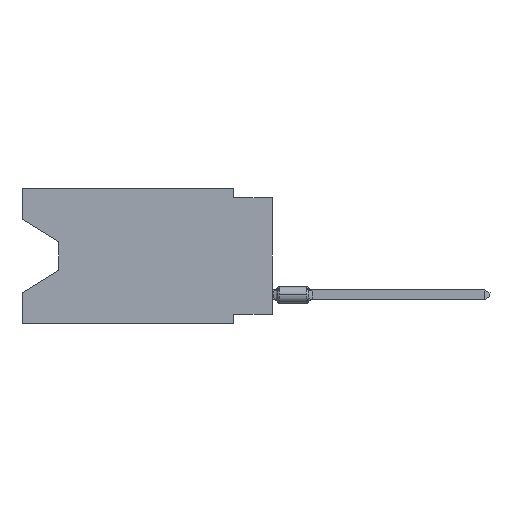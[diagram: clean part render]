
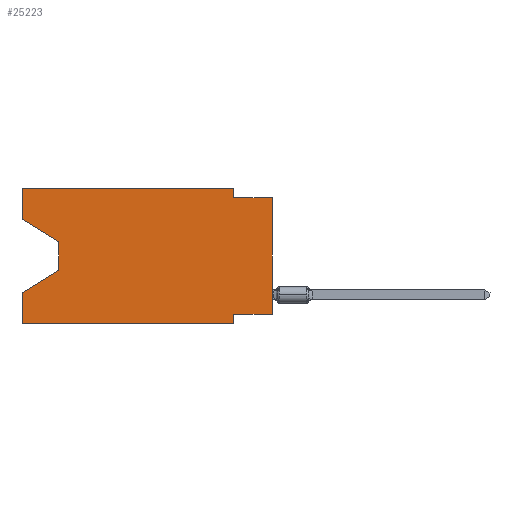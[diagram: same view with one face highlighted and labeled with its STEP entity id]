
A CAD part, left-side view. The second image highlights one B-rep face of the part: STEP entity #25223.
In plain terms, the highlighted planar face has unit normal (-1, 0, 0).
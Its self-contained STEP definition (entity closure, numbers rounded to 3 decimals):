
#1275 = EDGE_CURVE ( 'NONE', #24755, #3150, #7686, .T. ) ;
#1803 = CARTESIAN_POINT ( 'NONE',  ( 0., 16.383, -8.89 ) ) ;
#1833 = VECTOR ( 'NONE', #9087, 1000. ) ;
#2582 = VERTEX_POINT ( 'NONE', #27055 ) ;
#2785 = VECTOR ( 'NONE', #10349, 1000. ) ;
#3089 = EDGE_CURVE ( 'NONE', #15983, #5152, #23669, .T. ) ;
#3150 = VERTEX_POINT ( 'NONE', #28133 ) ;
#3367 = CARTESIAN_POINT ( 'NONE',  ( 0., 0., -8.255 ) ) ;
#3498 = DIRECTION ( 'NONE',  ( 0., 0., -1. ) ) ;
#3614 = EDGE_CURVE ( 'NONE', #11647, #7327, #6620, .T. ) ;
#3908 = ORIENTED_EDGE ( 'NONE', *, *, #19870, .F. ) ;
#3982 = EDGE_CURVE ( 'NONE', #15591, #26868, #17075, .T. ) ;
#4690 = EDGE_CURVE ( 'NONE', #2582, #9378, #27393, .T. ) ;
#5029 = CARTESIAN_POINT ( 'NONE',  ( 0., 13.97, -5.385 ) ) ;
#5152 = VERTEX_POINT ( 'NONE', #11889 ) ;
#5889 = VECTOR ( 'NONE', #22498, 1000. ) ;
#6497 = VECTOR ( 'NONE', #12562, 1000. ) ;
#6620 = LINE ( 'NONE', #26094, #10664 ) ;
#7010 = CARTESIAN_POINT ( 'NONE',  ( 0., 16.383, 0. ) ) ;
#7327 = VERTEX_POINT ( 'NONE', #7010 ) ;
#7686 = LINE ( 'NONE', #25552, #28311 ) ;
#8319 = CARTESIAN_POINT ( 'NONE',  ( 0., 16.383, 0. ) ) ;
#8460 = CARTESIAN_POINT ( 'NONE',  ( 0., 16.383, -8.89 ) ) ;
#9087 = DIRECTION ( 'NONE',  ( 0., -0.855, -0.519 ) ) ;
#9217 = CARTESIAN_POINT ( 'NONE',  ( 0., 16.383, -2.038 ) ) ;
#9378 = VERTEX_POINT ( 'NONE', #24182 ) ;
#9555 = ORIENTED_EDGE ( 'NONE', *, *, #1275, .F. ) ;
#9593 = DIRECTION ( 'NONE',  ( 0., 0., 1. ) ) ;
#9650 = CARTESIAN_POINT ( 'NONE',  ( 0., 16.383, 0. ) ) ;
#9838 = CARTESIAN_POINT ( 'NONE',  ( 0., 16.383, -2.038 ) ) ;
#10162 = DIRECTION ( 'NONE',  ( 0., 0.855, -0.519 ) ) ;
#10349 = DIRECTION ( 'NONE',  ( 0., -1., 0. ) ) ;
#10664 = VECTOR ( 'NONE', #17574, 1000. ) ;
#10940 = ORIENTED_EDGE ( 'NONE', *, *, #27351, .F. ) ;
#11150 = VECTOR ( 'NONE', #9593, 1000. ) ;
#11198 = CARTESIAN_POINT ( 'NONE',  ( 0., 13.97, -3.505 ) ) ;
#11403 = ORIENTED_EDGE ( 'NONE', *, *, #28469, .F. ) ;
#11463 = LINE ( 'NONE', #16072, #11150 ) ;
#11647 = VERTEX_POINT ( 'NONE', #9838 ) ;
#11766 = VECTOR ( 'NONE', #21712, 1000. ) ;
#11889 = CARTESIAN_POINT ( 'NONE',  ( 0., 0., -0.635 ) ) ;
#12340 = CARTESIAN_POINT ( 'NONE',  ( 0., 2.54, -8.255 ) ) ;
#12537 = VECTOR ( 'NONE', #21395, 1000. ) ;
#12562 = DIRECTION ( 'NONE',  ( 0., 0., 1. ) ) ;
#12809 = ORIENTED_EDGE ( 'NONE', *, *, #3614, .F. ) ;
#13126 = EDGE_CURVE ( 'NONE', #25447, #15591, #15209, .T. ) ;
#14466 = ORIENTED_EDGE ( 'NONE', *, *, #27129, .F. ) ;
#14626 = DIRECTION ( 'NONE',  ( 0., -1., 0. ) ) ;
#14767 = CARTESIAN_POINT ( 'NONE',  ( 0., 13.97, -5.385 ) ) ;
#14789 = CARTESIAN_POINT ( 'NONE',  ( 0., 16.383, -6.852 ) ) ;
#15209 = LINE ( 'NONE', #21575, #11766 ) ;
#15591 = VERTEX_POINT ( 'NONE', #5029 ) ;
#15708 = CARTESIAN_POINT ( 'NONE',  ( 0., 2.54, 0. ) ) ;
#15983 = VERTEX_POINT ( 'NONE', #3367 ) ;
#16072 = CARTESIAN_POINT ( 'NONE',  ( 0., 16.383, 0. ) ) ;
#16933 = LINE ( 'NONE', #22993, #12537 ) ;
#16954 = LINE ( 'NONE', #9650, #18618 ) ;
#17075 = LINE ( 'NONE', #14767, #20828 ) ;
#17118 = DIRECTION ( 'NONE',  ( 0., 0., -1. ) ) ;
#17268 = DIRECTION ( 'NONE',  ( 1., 0., 0. ) ) ;
#17574 = DIRECTION ( 'NONE',  ( 0., 0., 1. ) ) ;
#17654 = VERTEX_POINT ( 'NONE', #1803 ) ;
#18046 = ORIENTED_EDGE ( 'NONE', *, *, #3982, .T. ) ;
#18618 = VECTOR ( 'NONE', #20620, 1000. ) ;
#19297 = FACE_OUTER_BOUND ( 'NONE', #21103, .T. ) ;
#19500 = VECTOR ( 'NONE', #14626, 1000. ) ;
#19609 = ORIENTED_EDGE ( 'NONE', *, *, #23515, .T. ) ;
#19870 = EDGE_CURVE ( 'NONE', #7327, #2582, #16954, .T. ) ;
#20620 = DIRECTION ( 'NONE',  ( 0., -1., 0. ) ) ;
#20828 = VECTOR ( 'NONE', #10162, 1000. ) ;
#21103 = EDGE_LOOP ( 'NONE', ( #26978, #26921, #18046, #14466, #19609, #9555, #10940, #28236, #11403, #23524, #3908, #12809 ) ) ;
#21395 = DIRECTION ( 'NONE',  ( 0., 1., 0. ) ) ;
#21575 = CARTESIAN_POINT ( 'NONE',  ( 0., 13.97, -3.505 ) ) ;
#21712 = DIRECTION ( 'NONE',  ( 0., 0., -1. ) ) ;
#21728 = LINE ( 'NONE', #8460, #2785 ) ;
#22498 = DIRECTION ( 'NONE',  ( 0., 0., -1. ) ) ;
#22993 = CARTESIAN_POINT ( 'NONE',  ( 0., 0., -8.255 ) ) ;
#23287 = LINE ( 'NONE', #23420, #19500 ) ;
#23420 = CARTESIAN_POINT ( 'NONE',  ( 0., 0., -0.635 ) ) ;
#23515 = EDGE_CURVE ( 'NONE', #17654, #3150, #21728, .T. ) ;
#23524 = ORIENTED_EDGE ( 'NONE', *, *, #4690, .F. ) ;
#23669 = LINE ( 'NONE', #25558, #6497 ) ;
#24182 = CARTESIAN_POINT ( 'NONE',  ( 0., 2.54, -0.635 ) ) ;
#24634 = EDGE_CURVE ( 'NONE', #11647, #25447, #26670, .T. ) ;
#24755 = VERTEX_POINT ( 'NONE', #12340 ) ;
#25223 = ADVANCED_FACE ( 'NONE', ( #19297 ), #28076, .F. ) ;
#25447 = VERTEX_POINT ( 'NONE', #11198 ) ;
#25552 = CARTESIAN_POINT ( 'NONE',  ( 0., 2.54, -8.89 ) ) ;
#25558 = CARTESIAN_POINT ( 'NONE',  ( 0., 0., 0. ) ) ;
#26094 = CARTESIAN_POINT ( 'NONE',  ( 0., 16.383, 0. ) ) ;
#26670 = LINE ( 'NONE', #9217, #1833 ) ;
#26868 = VERTEX_POINT ( 'NONE', #14789 ) ;
#26921 = ORIENTED_EDGE ( 'NONE', *, *, #13126, .T. ) ;
#26978 = ORIENTED_EDGE ( 'NONE', *, *, #24634, .T. ) ;
#27055 = CARTESIAN_POINT ( 'NONE',  ( 0., 2.54, 0. ) ) ;
#27129 = EDGE_CURVE ( 'NONE', #17654, #26868, #11463, .T. ) ;
#27203 = AXIS2_PLACEMENT_3D ( 'NONE', #8319, #17268, #17118 ) ;
#27351 = EDGE_CURVE ( 'NONE', #15983, #24755, #16933, .T. ) ;
#27393 = LINE ( 'NONE', #15708, #5889 ) ;
#28076 = PLANE ( 'NONE',  #27203 ) ;
#28133 = CARTESIAN_POINT ( 'NONE',  ( 0., 2.54, -8.89 ) ) ;
#28236 = ORIENTED_EDGE ( 'NONE', *, *, #3089, .T. ) ;
#28311 = VECTOR ( 'NONE', #3498, 1000. ) ;
#28469 = EDGE_CURVE ( 'NONE', #9378, #5152, #23287, .T. ) ;
